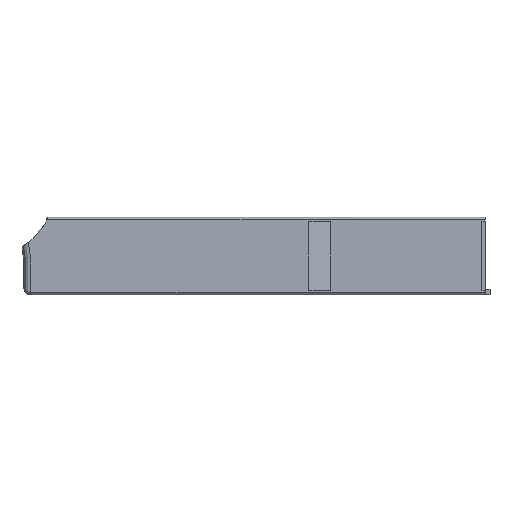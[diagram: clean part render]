
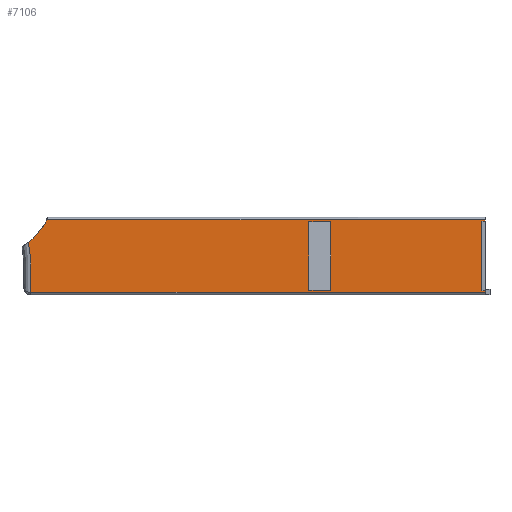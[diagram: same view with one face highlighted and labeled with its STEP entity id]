
A CAD part, left-side view. The second image highlights one B-rep face of the part: STEP entity #7106.
In plain terms, the highlighted planar face has unit normal (-1, 0, 0).
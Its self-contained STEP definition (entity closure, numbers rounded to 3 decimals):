
#23 = DIRECTION ( 'NONE',  ( 0., -0.281, 0.96 ) ) ;
#206 = VERTEX_POINT ( 'NONE', #4224 ) ;
#216 = VECTOR ( 'NONE', #857, 1000. ) ;
#242 = VERTEX_POINT ( 'NONE', #3243 ) ;
#326 = VERTEX_POINT ( 'NONE', #3441 ) ;
#344 = ORIENTED_EDGE ( 'NONE', *, *, #8687, .F. ) ;
#350 = VERTEX_POINT ( 'NONE', #11674 ) ;
#509 = VECTOR ( 'NONE', #4682, 1000. ) ;
#522 = DIRECTION ( 'NONE',  ( 0., 0., -1. ) ) ;
#536 = PLANE ( 'NONE',  #9172 ) ;
#547 = CARTESIAN_POINT ( 'NONE',  ( -10.5, 197.568, 2.355 ) ) ;
#787 = VECTOR ( 'NONE', #3745, 1000. ) ;
#857 = DIRECTION ( 'NONE',  ( 0., 1., 0. ) ) ;
#951 = EDGE_CURVE ( 'NONE', #8988, #242, #8537, .T. ) ;
#965 = CARTESIAN_POINT ( 'NONE',  ( -10.5, 1.5, -15.05 ) ) ;
#998 = EDGE_LOOP ( 'NONE', ( #6460, #4414, #4936, #4443 ) ) ;
#1196 = VERTEX_POINT ( 'NONE', #11639 ) ;
#1332 = CARTESIAN_POINT ( 'NONE',  ( -10.5, 0., -15.75 ) ) ;
#1452 = CARTESIAN_POINT ( 'NONE',  ( -10.5, 197.187, -0.341 ) ) ;
#1498 = VERTEX_POINT ( 'NONE', #10043 ) ;
#1514 = VERTEX_POINT ( 'NONE', #8330 ) ;
#1586 = CARTESIAN_POINT ( 'NONE',  ( -10.5, 76.5, 14.75 ) ) ;
#1610 = EDGE_CURVE ( 'NONE', #7908, #1514, #5826, .T. ) ;
#1666 = EDGE_CURVE ( 'NONE', #326, #11715, #3161, .T. ) ;
#1704 = CARTESIAN_POINT ( 'NONE',  ( -10.5, 76.5, -14.75 ) ) ;
#1808 = VECTOR ( 'NONE', #6315, 1000. ) ;
#2128 = CARTESIAN_POINT ( 'NONE',  ( -10.5, 1.5, 15.05 ) ) ;
#2235 = EDGE_CURVE ( 'NONE', #206, #350, #3081, .T. ) ;
#2305 = VECTOR ( 'NONE', #3350, 1000. ) ;
#2378 = CARTESIAN_POINT ( 'NONE',  ( -10.5, 196.988, -2.597 ) ) ;
#2766 = ORIENTED_EDGE ( 'NONE', *, *, #6827, .T. ) ;
#2803 = CARTESIAN_POINT ( 'NONE',  ( -10.5, 200., -15.75 ) ) ;
#2822 = VERTEX_POINT ( 'NONE', #6425 ) ;
#2869 = LINE ( 'NONE', #10543, #2305 ) ;
#2928 = LINE ( 'NONE', #3792, #509 ) ;
#2946 = VECTOR ( 'NONE', #3691, 1000. ) ;
#3081 = B_SPLINE_CURVE_WITH_KNOTS ( 'NONE', 3,
 ( #5593, #4123, #5947, #547, #6852, #1452, #7774, #2378, #8664, #3283, #9574, #4157, #10475, #5071, #11382, #5978 ),
 .UNSPECIFIED., .F., .F.,
 ( 4, 2, 2, 2, 2, 2, 2, 4 ),
 ( 0., 0.003, 0.005, 0.008, 0.01, 0.011, 0.016, 0.022 ),
 .UNSPECIFIED. ) ;
#3097 = EDGE_CURVE ( 'NONE', #5411, #1514, #3164, .T. ) ;
#3161 = LINE ( 'NONE', #7718, #5540 ) ;
#3164 = LINE ( 'NONE', #7342, #9483 ) ;
#3243 = CARTESIAN_POINT ( 'NONE',  ( -10.5, 190.111, 15.75 ) ) ;
#3274 = DIRECTION ( 'NONE',  ( 0., 0., 1. ) ) ;
#3283 = CARTESIAN_POINT ( 'NONE',  ( -10.5, 196.964, -3.957 ) ) ;
#3350 = DIRECTION ( 'NONE',  ( 0., 0., -1. ) ) ;
#3441 = CARTESIAN_POINT ( 'NONE',  ( -10.5, 196.991, -15.75 ) ) ;
#3676 = CARTESIAN_POINT ( 'NONE',  ( -10.5, 202.161, 2.879 ) ) ;
#3691 = DIRECTION ( 'NONE',  ( 0., -1., 0. ) ) ;
#3738 = VECTOR ( 'NONE', #23, 1000. ) ;
#3745 = DIRECTION ( 'NONE',  ( 0., -1., 0. ) ) ;
#3767 = EDGE_LOOP ( 'NONE', ( #11632, #10389, #4699, #8730, #6265, #344, #9538, #6281, #3888, #2766, #4042, #8316 ) ) ;
#3783 = LINE ( 'NONE', #1586, #5899 ) ;
#3792 = CARTESIAN_POINT ( 'NONE',  ( -10.5, 0., 0. ) ) ;
#3888 = ORIENTED_EDGE ( 'NONE', *, *, #3097, .F. ) ;
#3944 = CARTESIAN_POINT ( 'NONE',  ( -10.5, 67., -14.75 ) ) ;
#4000 = EDGE_CURVE ( 'NONE', #7908, #1498, #2869, .T. ) ;
#4042 = ORIENTED_EDGE ( 'NONE', *, *, #951, .F. ) ;
#4123 = CARTESIAN_POINT ( 'NONE',  ( -10.5, 197.945, 5.052 ) ) ;
#4157 = CARTESIAN_POINT ( 'NONE',  ( -10.5, 196.96, -6.678 ) ) ;
#4205 = DIRECTION ( 'NONE',  ( 0., -0.636, 0.771 ) ) ;
#4224 = CARTESIAN_POINT ( 'NONE',  ( -10.5, 198.068, 5.951 ) ) ;
#4414 = ORIENTED_EDGE ( 'NONE', *, *, #11202, .F. ) ;
#4423 = VECTOR ( 'NONE', #8175, 1000. ) ;
#4443 = ORIENTED_EDGE ( 'NONE', *, *, #10536, .T. ) ;
#4566 = DIRECTION ( 'NONE',  ( 0., -0.8, 0.6 ) ) ;
#4682 = DIRECTION ( 'NONE',  ( 0., 0., -1. ) ) ;
#4699 = ORIENTED_EDGE ( 'NONE', *, *, #5746, .T. ) ;
#4711 = EDGE_CURVE ( 'NONE', #1196, #2822, #3783, .T. ) ;
#4740 = VECTOR ( 'NONE', #4205, 1000. ) ;
#4789 = VERTEX_POINT ( 'NONE', #8841 ) ;
#4936 = ORIENTED_EDGE ( 'NONE', *, *, #4711, .F. ) ;
#5003 = CARTESIAN_POINT ( 'NONE',  ( -10.5, 67., 26.458 ) ) ;
#5071 = CARTESIAN_POINT ( 'NONE',  ( -10.5, 196.985, -12.121 ) ) ;
#5286 = LINE ( 'NONE', #9128, #787 ) ;
#5393 = CARTESIAN_POINT ( 'NONE',  ( -10.5, 76.5, 26.458 ) ) ;
#5411 = VERTEX_POINT ( 'NONE', #7498 ) ;
#5540 = VECTOR ( 'NONE', #8578, 1000. ) ;
#5593 = CARTESIAN_POINT ( 'NONE',  ( -10.5, 198.068, 5.951 ) ) ;
#5606 = LINE ( 'NONE', #2803, #2946 ) ;
#5733 = FACE_OUTER_BOUND ( 'NONE', #3767, .T. ) ;
#5746 = EDGE_CURVE ( 'NONE', #350, #326, #5606, .T. ) ;
#5826 = LINE ( 'NONE', #2128, #10336 ) ;
#5899 = VECTOR ( 'NONE', #9706, 1000. ) ;
#5947 = CARTESIAN_POINT ( 'NONE',  ( -10.5, 197.821, 4.152 ) ) ;
#5978 = CARTESIAN_POINT ( 'NONE',  ( -10.5, 196.997, -15.75 ) ) ;
#6189 = VERTEX_POINT ( 'NONE', #1704 ) ;
#6244 = VECTOR ( 'NONE', #522, 1000. ) ;
#6265 = ORIENTED_EDGE ( 'NONE', *, *, #6622, .F. ) ;
#6281 = ORIENTED_EDGE ( 'NONE', *, *, #1610, .T. ) ;
#6315 = DIRECTION ( 'NONE',  ( 0., 0., -1. ) ) ;
#6360 = CARTESIAN_POINT ( 'NONE',  ( -10.5, 195.137, -1.423 ) ) ;
#6425 = CARTESIAN_POINT ( 'NONE',  ( -10.5, 76.5, 14.75 ) ) ;
#6460 = ORIENTED_EDGE ( 'NONE', *, *, #6614, .F. ) ;
#6552 = LINE ( 'NONE', #5003, #6244 ) ;
#6614 = EDGE_CURVE ( 'NONE', #6189, #10919, #5286, .T. ) ;
#6622 = EDGE_CURVE ( 'NONE', #7097, #11715, #2928, .T. ) ;
#6768 = EDGE_CURVE ( 'NONE', #4789, #8988, #9235, .T. ) ;
#6827 = EDGE_CURVE ( 'NONE', #5411, #242, #8952, .T. ) ;
#6838 = CARTESIAN_POINT ( 'NONE',  ( -10.5, 0., -15.05 ) ) ;
#6844 = LINE ( 'NONE', #965, #4423 ) ;
#6852 = CARTESIAN_POINT ( 'NONE',  ( -10.5, 197.437, 1.457 ) ) ;
#7097 = VERTEX_POINT ( 'NONE', #6838 ) ;
#7106 = ADVANCED_FACE ( 'NONE', ( #7852, #5733 ), #536, .T. ) ;
#7342 = CARTESIAN_POINT ( 'NONE',  ( -10.5, 0., 0. ) ) ;
#7418 = LINE ( 'NONE', #3676, #8947 ) ;
#7498 = CARTESIAN_POINT ( 'NONE',  ( -10.5, 0., 15.75 ) ) ;
#7718 = CARTESIAN_POINT ( 'NONE',  ( -10.5, 200., -15.75 ) ) ;
#7763 = CARTESIAN_POINT ( 'NONE',  ( -10.5, 200., 0. ) ) ;
#7774 = CARTESIAN_POINT ( 'NONE',  ( -10.5, 197.068, -1.241 ) ) ;
#7852 = FACE_BOUND ( 'NONE', #998, .T. ) ;
#7908 = VERTEX_POINT ( 'NONE', #10378 ) ;
#8175 = DIRECTION ( 'NONE',  ( 0., -1., 0. ) ) ;
#8255 = DIRECTION ( 'NONE',  ( 0., 0., -1. ) ) ;
#8316 = ORIENTED_EDGE ( 'NONE', *, *, #6768, .F. ) ;
#8330 = CARTESIAN_POINT ( 'NONE',  ( -10.5, 0., 15.05 ) ) ;
#8429 = DIRECTION ( 'NONE',  ( 0., -1., 0. ) ) ;
#8537 = LINE ( 'NONE', #6360, #3738 ) ;
#8578 = DIRECTION ( 'NONE',  ( 0., -1., 0. ) ) ;
#8655 = DIRECTION ( 'NONE',  ( -1., 0., 0. ) ) ;
#8664 = CARTESIAN_POINT ( 'NONE',  ( -10.5, 196.977, -3.05 ) ) ;
#8687 = EDGE_CURVE ( 'NONE', #1498, #7097, #6844, .T. ) ;
#8718 = LINE ( 'NONE', #5393, #1808 ) ;
#8721 = EDGE_CURVE ( 'NONE', #206, #4789, #7418, .T. ) ;
#8730 = ORIENTED_EDGE ( 'NONE', *, *, #1666, .T. ) ;
#8841 = CARTESIAN_POINT ( 'NONE',  ( -10.5, 196., 7.503 ) ) ;
#8947 = VECTOR ( 'NONE', #4566, 1000. ) ;
#8952 = LINE ( 'NONE', #11653, #216 ) ;
#8988 = VERTEX_POINT ( 'NONE', #10903 ) ;
#9128 = CARTESIAN_POINT ( 'NONE',  ( -10.5, 76.5, -14.75 ) ) ;
#9172 = AXIS2_PLACEMENT_3D ( 'NONE', #7763, #8655, #3274 ) ;
#9235 = LINE ( 'NONE', #10662, #4740 ) ;
#9483 = VECTOR ( 'NONE', #8255, 1000. ) ;
#9538 = ORIENTED_EDGE ( 'NONE', *, *, #4000, .F. ) ;
#9574 = CARTESIAN_POINT ( 'NONE',  ( -10.5, 196.963, -4.41 ) ) ;
#9706 = DIRECTION ( 'NONE',  ( 0., 1., 0. ) ) ;
#10043 = CARTESIAN_POINT ( 'NONE',  ( -10.5, 1.5, -15.05 ) ) ;
#10336 = VECTOR ( 'NONE', #8429, 1000. ) ;
#10378 = CARTESIAN_POINT ( 'NONE',  ( -10.5, 1.5, 15.05 ) ) ;
#10389 = ORIENTED_EDGE ( 'NONE', *, *, #2235, .T. ) ;
#10475 = CARTESIAN_POINT ( 'NONE',  ( -10.5, 196.971, -8.493 ) ) ;
#10536 = EDGE_CURVE ( 'NONE', #1196, #10919, #6552, .T. ) ;
#10543 = CARTESIAN_POINT ( 'NONE',  ( -10.5, 1.5, 0. ) ) ;
#10662 = CARTESIAN_POINT ( 'NONE',  ( -10.5, 201.302, 1.074 ) ) ;
#10903 = CARTESIAN_POINT ( 'NONE',  ( -10.5, 190.613, 14.036 ) ) ;
#10919 = VERTEX_POINT ( 'NONE', #3944 ) ;
#11202 = EDGE_CURVE ( 'NONE', #2822, #6189, #8718, .T. ) ;
#11382 = CARTESIAN_POINT ( 'NONE',  ( -10.5, 196.992, -13.936 ) ) ;
#11632 = ORIENTED_EDGE ( 'NONE', *, *, #8721, .F. ) ;
#11639 = CARTESIAN_POINT ( 'NONE',  ( -10.5, 67., 14.75 ) ) ;
#11653 = CARTESIAN_POINT ( 'NONE',  ( -10.5, 189.818, 15.75 ) ) ;
#11674 = CARTESIAN_POINT ( 'NONE',  ( -10.5, 196.997, -15.75 ) ) ;
#11715 = VERTEX_POINT ( 'NONE', #1332 ) ;
